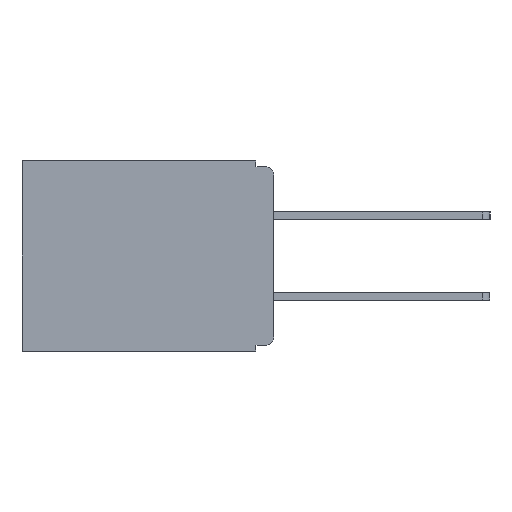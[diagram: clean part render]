
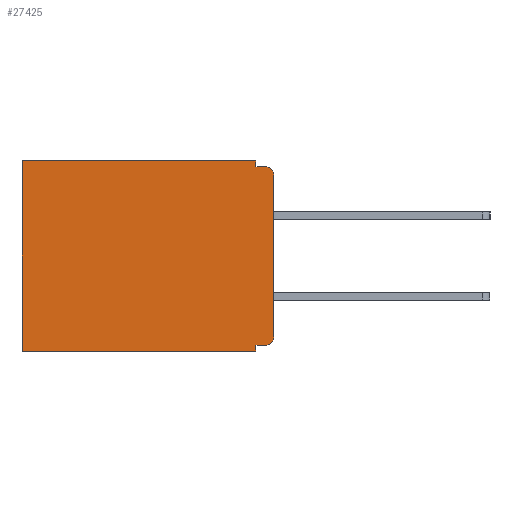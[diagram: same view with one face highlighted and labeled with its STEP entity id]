
A CAD part, left-side view. The second image highlights one B-rep face of the part: STEP entity #27425.
In plain terms, the highlighted planar face has unit normal (-1, 0, 0).
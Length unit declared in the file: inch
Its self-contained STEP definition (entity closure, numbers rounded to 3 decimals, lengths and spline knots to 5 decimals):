
#640 = EDGE_CURVE ( 'NONE', #16925, #29098, #749, .T. ) ;
#749 = LINE ( 'NONE', #22075, #13439 ) ;
#888 = ORIENTED_EDGE ( 'NONE', *, *, #19905, .F. ) ;
#1790 = VERTEX_POINT ( 'NONE', #25179 ) ;
#2896 = CARTESIAN_POINT ( 'NONE',  ( 0.3, 0.015, -0.025 ) ) ;
#3385 = LINE ( 'NONE', #21054, #16126 ) ;
#3597 = EDGE_CURVE ( 'NONE', #9789, #21457, #10959, .T. ) ;
#3645 = CARTESIAN_POINT ( 'NONE',  ( 0.3, 0., -0.32 ) ) ;
#3838 = VERTEX_POINT ( 'NONE', #15133 ) ;
#4274 = AXIS2_PLACEMENT_3D ( 'NONE', #10450, #27812, #12968 ) ;
#4591 = ORIENTED_EDGE ( 'NONE', *, *, #22877, .T. ) ;
#4714 = VERTEX_POINT ( 'NONE', #26163 ) ;
#4902 = DIRECTION ( 'NONE',  ( 0., 0., -1. ) ) ;
#5013 = CARTESIAN_POINT ( 'NONE',  ( 0.3, 0.031, 0. ) ) ;
#5095 = CARTESIAN_POINT ( 'NONE',  ( 0.3, 0., -0.01 ) ) ;
#5286 = CARTESIAN_POINT ( 'NONE',  ( 0.3, 0.015, -0.32 ) ) ;
#5489 = DIRECTION ( 'NONE',  ( 0., 0., -1. ) ) ;
#6687 = EDGE_LOOP ( 'NONE', ( #23393, #4591, #14019, #888, #8749, #18418, #10938, #20280, #28286, #30984 ) ) ;
#6759 = VECTOR ( 'NONE', #21095, 39.37008 ) ;
#6809 = DIRECTION ( 'NONE',  ( 0., 1., 0. ) ) ;
#6956 = DIRECTION ( 'NONE',  ( 0., 0., -1. ) ) ;
#7561 = CARTESIAN_POINT ( 'NONE',  ( 0.3, 0.031, 0. ) ) ;
#8631 = CIRCLE ( 'NONE', #4274, 0.015 ) ;
#8749 = ORIENTED_EDGE ( 'NONE', *, *, #15467, .T. ) ;
#9789 = VERTEX_POINT ( 'NONE', #5286 ) ;
#9912 = EDGE_CURVE ( 'NONE', #11953, #4714, #24187, .T. ) ;
#10450 = CARTESIAN_POINT ( 'NONE',  ( 0.3, 0.015, -0.305 ) ) ;
#10938 = ORIENTED_EDGE ( 'NONE', *, *, #17609, .F. ) ;
#10959 = LINE ( 'NONE', #3645, #23435 ) ;
#11082 = CARTESIAN_POINT ( 'NONE',  ( 0.3, 0., 0. ) ) ;
#11649 = DIRECTION ( 'NONE',  ( 0., 0., -1. ) ) ;
#11953 = VERTEX_POINT ( 'NONE', #21265 ) ;
#12506 = AXIS2_PLACEMENT_3D ( 'NONE', #2896, #20585, #5489 ) ;
#12846 = EDGE_CURVE ( 'NONE', #9789, #4714, #8631, .T. ) ;
#12968 = DIRECTION ( 'NONE',  ( 0., 0., -1. ) ) ;
#13217 = EDGE_CURVE ( 'NONE', #21457, #1790, #29884, .T. ) ;
#13432 = DIRECTION ( 'NONE',  ( 0., 0., -1. ) ) ;
#13439 = VECTOR ( 'NONE', #16207, 39.37008 ) ;
#14019 = ORIENTED_EDGE ( 'NONE', *, *, #27187, .F. ) ;
#15133 = CARTESIAN_POINT ( 'NONE',  ( 0.3, 0.031, -0.01 ) ) ;
#15467 = EDGE_CURVE ( 'NONE', #24762, #16925, #26705, .T. ) ;
#16126 = VECTOR ( 'NONE', #16144, 39.37008 ) ;
#16144 = DIRECTION ( 'NONE',  ( 0., 1., 0. ) ) ;
#16207 = DIRECTION ( 'NONE',  ( 0., 0., -1. ) ) ;
#16925 = VERTEX_POINT ( 'NONE', #20535 ) ;
#17558 = VECTOR ( 'NONE', #6956, 39.37008 ) ;
#17609 = EDGE_CURVE ( 'NONE', #1790, #29098, #3385, .T. ) ;
#18418 = ORIENTED_EDGE ( 'NONE', *, *, #640, .T. ) ;
#18737 = FACE_OUTER_BOUND ( 'NONE', #6687, .T. ) ;
#19905 = EDGE_CURVE ( 'NONE', #24762, #3838, #26658, .T. ) ;
#20280 = ORIENTED_EDGE ( 'NONE', *, *, #13217, .F. ) ;
#20535 = CARTESIAN_POINT ( 'NONE',  ( 0.3, 0.437, 0. ) ) ;
#20585 = DIRECTION ( 'NONE',  ( -1., 0., 0. ) ) ;
#21054 = CARTESIAN_POINT ( 'NONE',  ( 0.3, 0., -0.33 ) ) ;
#21095 = DIRECTION ( 'NONE',  ( 0., 1., 0. ) ) ;
#21265 = CARTESIAN_POINT ( 'NONE',  ( 0.3, 0., -0.025 ) ) ;
#21457 = VERTEX_POINT ( 'NONE', #27156 ) ;
#21558 = PLANE ( 'NONE',  #24725 ) ;
#22013 = CARTESIAN_POINT ( 'NONE',  ( 0.3, 0.031, -0.33 ) ) ;
#22075 = CARTESIAN_POINT ( 'NONE',  ( 0.3, 0.437, -0.33 ) ) ;
#22754 = DIRECTION ( 'NONE',  ( 0., -1., 0. ) ) ;
#22877 = EDGE_CURVE ( 'NONE', #11953, #23141, #29182, .T. ) ;
#23141 = VERTEX_POINT ( 'NONE', #31362 ) ;
#23393 = ORIENTED_EDGE ( 'NONE', *, *, #9912, .F. ) ;
#23435 = VECTOR ( 'NONE', #6809, 39.37008 ) ;
#24048 = CARTESIAN_POINT ( 'NONE',  ( 0.3, 0., -0.33 ) ) ;
#24187 = LINE ( 'NONE', #28272, #31360 ) ;
#24207 = LINE ( 'NONE', #5095, #30617 ) ;
#24725 = AXIS2_PLACEMENT_3D ( 'NONE', #24048, #26493, #11649 ) ;
#24762 = VERTEX_POINT ( 'NONE', #5013 ) ;
#25179 = CARTESIAN_POINT ( 'NONE',  ( 0.3, 0.031, -0.33 ) ) ;
#26163 = CARTESIAN_POINT ( 'NONE',  ( 0.3, 0., -0.305 ) ) ;
#26493 = DIRECTION ( 'NONE',  ( 1., 0., 0. ) ) ;
#26658 = LINE ( 'NONE', #7561, #31543 ) ;
#26705 = LINE ( 'NONE', #11082, #6759 ) ;
#27156 = CARTESIAN_POINT ( 'NONE',  ( 0.3, 0.031, -0.32 ) ) ;
#27187 = EDGE_CURVE ( 'NONE', #3838, #23141, #24207, .T. ) ;
#27425 = ADVANCED_FACE ( 'NONE', ( #18737 ), #21558, .F. ) ;
#27812 = DIRECTION ( 'NONE',  ( -1., 0., 0. ) ) ;
#28096 = CARTESIAN_POINT ( 'NONE',  ( 0.3, 0.437, -0.33 ) ) ;
#28272 = CARTESIAN_POINT ( 'NONE',  ( 0.3, 0., -0.33 ) ) ;
#28286 = ORIENTED_EDGE ( 'NONE', *, *, #3597, .F. ) ;
#29098 = VERTEX_POINT ( 'NONE', #28096 ) ;
#29182 = CIRCLE ( 'NONE', #12506, 0.015 ) ;
#29884 = LINE ( 'NONE', #22013, #17558 ) ;
#30617 = VECTOR ( 'NONE', #22754, 39.37008 ) ;
#30984 = ORIENTED_EDGE ( 'NONE', *, *, #12846, .T. ) ;
#31360 = VECTOR ( 'NONE', #13432, 39.37008 ) ;
#31362 = CARTESIAN_POINT ( 'NONE',  ( 0.3, 0.015, -0.01 ) ) ;
#31543 = VECTOR ( 'NONE', #4902, 39.37008 ) ;
